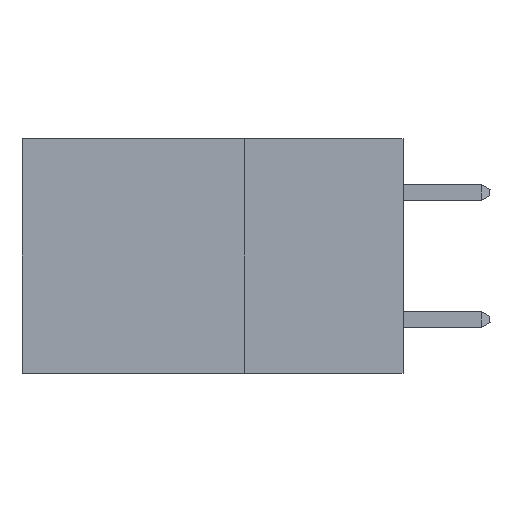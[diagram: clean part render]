
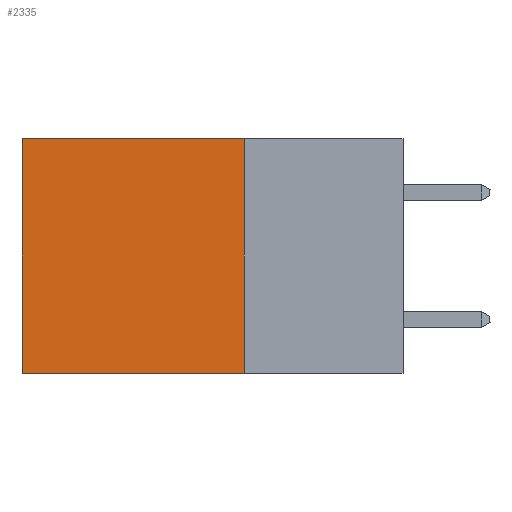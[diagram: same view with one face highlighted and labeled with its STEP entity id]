
A CAD part, left-side view. The second image highlights one B-rep face of the part: STEP entity #2335.
In plain terms, the highlighted planar face has unit normal (-1, 0, 0).
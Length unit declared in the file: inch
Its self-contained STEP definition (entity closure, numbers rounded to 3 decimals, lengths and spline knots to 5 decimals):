
#345 = DIRECTION ( 'NONE',  ( 0., 1., 0. ) ) ;
#548 = VERTEX_POINT ( 'NONE', #4720 ) ;
#1015 = FACE_OUTER_BOUND ( 'NONE', #1048, .T. ) ;
#1048 = EDGE_LOOP ( 'NONE', ( #6036, #7970, #6284, #8203 ) ) ;
#1839 = CARTESIAN_POINT ( 'NONE',  ( 0.2875, 0.6, 0. ) ) ;
#2335 = ADVANCED_FACE ( 'NONE', ( #1015 ), #6748, .F. ) ;
#2429 = DIRECTION ( 'NONE',  ( 0., 1., 0. ) ) ;
#2610 = DIRECTION ( 'NONE',  ( 0., 0., -1. ) ) ;
#3062 = CARTESIAN_POINT ( 'NONE',  ( 0.2875, 0.25, -0.37 ) ) ;
#3315 = CARTESIAN_POINT ( 'NONE',  ( 0.2875, 0.25, 0. ) ) ;
#3795 = VECTOR ( 'NONE', #2429, 39.37008 ) ;
#4613 = VECTOR ( 'NONE', #345, 39.37008 ) ;
#4720 = CARTESIAN_POINT ( 'NONE',  ( 0.2875, 0.25, 0. ) ) ;
#4762 = DIRECTION ( 'NONE',  ( 0., 0., -1. ) ) ;
#5050 = LINE ( 'NONE', #3062, #4613 ) ;
#5087 = EDGE_CURVE ( 'NONE', #8554, #8470, #8704, .T. ) ;
#5323 = CARTESIAN_POINT ( 'NONE',  ( 0.2875, 0.25, 0. ) ) ;
#5702 = LINE ( 'NONE', #5323, #3795 ) ;
#6036 = ORIENTED_EDGE ( 'NONE', *, *, #5087, .T. ) ;
#6212 = CARTESIAN_POINT ( 'NONE',  ( 0.2875, 0.6, 0. ) ) ;
#6273 = EDGE_CURVE ( 'NONE', #7960, #8470, #5050, .T. ) ;
#6284 = ORIENTED_EDGE ( 'NONE', *, *, #9282, .F. ) ;
#6615 = DIRECTION ( 'NONE',  ( 0., 0., -1. ) ) ;
#6625 = DIRECTION ( 'NONE',  ( 1., 0., 0. ) ) ;
#6677 = CARTESIAN_POINT ( 'NONE',  ( 0.2875, 0.25, 0. ) ) ;
#6748 = PLANE ( 'NONE',  #8786 ) ;
#6830 = VECTOR ( 'NONE', #2610, 39.37008 ) ;
#6869 = LINE ( 'NONE', #3315, #8532 ) ;
#7580 = CARTESIAN_POINT ( 'NONE',  ( 0.2875, 0.6, -0.37 ) ) ;
#7960 = VERTEX_POINT ( 'NONE', #8569 ) ;
#7970 = ORIENTED_EDGE ( 'NONE', *, *, #6273, .F. ) ;
#8203 = ORIENTED_EDGE ( 'NONE', *, *, #8416, .T. ) ;
#8416 = EDGE_CURVE ( 'NONE', #548, #8554, #5702, .T. ) ;
#8470 = VERTEX_POINT ( 'NONE', #7580 ) ;
#8532 = VECTOR ( 'NONE', #4762, 39.37008 ) ;
#8554 = VERTEX_POINT ( 'NONE', #1839 ) ;
#8569 = CARTESIAN_POINT ( 'NONE',  ( 0.2875, 0.25, -0.37 ) ) ;
#8704 = LINE ( 'NONE', #6212, #6830 ) ;
#8786 = AXIS2_PLACEMENT_3D ( 'NONE', #6677, #6625, #6615 ) ;
#9282 = EDGE_CURVE ( 'NONE', #548, #7960, #6869, .T. ) ;
